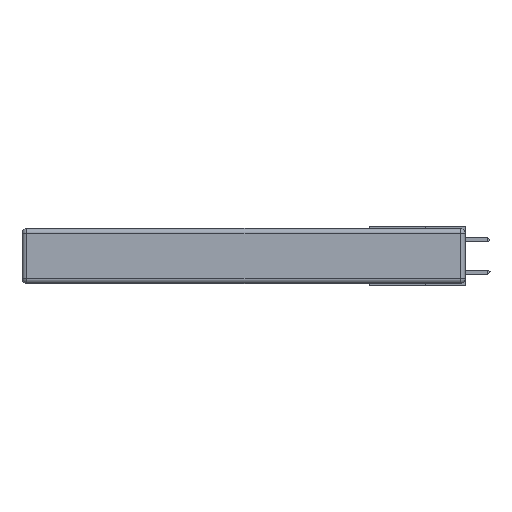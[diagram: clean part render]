
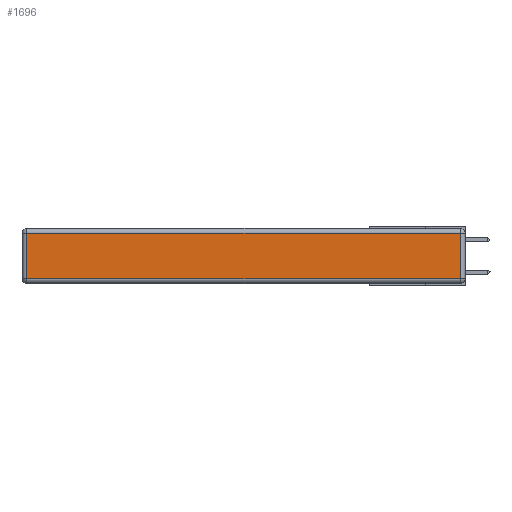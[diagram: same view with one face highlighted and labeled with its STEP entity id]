
A CAD part, left-side view. The second image highlights one B-rep face of the part: STEP entity #1696.
In plain terms, the highlighted planar face has unit normal (-1, 0, 0).
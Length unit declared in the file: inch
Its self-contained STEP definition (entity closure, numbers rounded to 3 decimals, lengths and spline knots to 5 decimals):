
#2 = DIRECTION ( 'NONE',  ( 0., 0., 1. ) ) ;
#451 = EDGE_CURVE ( 'NONE', #13760, #1633, #15265, .T. ) ;
#570 = LINE ( 'NONE', #2552, #5573 ) ;
#1633 = VERTEX_POINT ( 'NONE', #9276 ) ;
#1685 = DIRECTION ( 'NONE',  ( 0., -1., 0. ) ) ;
#1696 = ADVANCED_FACE ( 'NONE', ( #8168 ), #12979, .T. ) ;
#2439 = LINE ( 'NONE', #14198, #6668 ) ;
#2552 = CARTESIAN_POINT ( 'NONE',  ( 0., 2.72, -0.343 ) ) ;
#2918 = DIRECTION ( 'NONE',  ( 0., 1., 0. ) ) ;
#3330 = VERTEX_POINT ( 'NONE', #6634 ) ;
#5093 = LINE ( 'NONE', #8690, #9300 ) ;
#5573 = VECTOR ( 'NONE', #8496, 39.37008 ) ;
#5668 = EDGE_CURVE ( 'NONE', #1633, #10206, #2439, .T. ) ;
#5844 = DIRECTION ( 'NONE',  ( -1., 0., 0. ) ) ;
#6055 = ORIENTED_EDGE ( 'NONE', *, *, #5668, .T. ) ;
#6084 = EDGE_LOOP ( 'NONE', ( #11812, #6055, #13515, #13216 ) ) ;
#6634 = CARTESIAN_POINT ( 'NONE',  ( 0., 2.72, -0.03 ) ) ;
#6668 = VECTOR ( 'NONE', #7100, 39.37008 ) ;
#7100 = DIRECTION ( 'NONE',  ( 0., 0., 1. ) ) ;
#8168 = FACE_OUTER_BOUND ( 'NONE', #6084, .T. ) ;
#8496 = DIRECTION ( 'NONE',  ( 0., 0., -1. ) ) ;
#8575 = VECTOR ( 'NONE', #1685, 39.37008 ) ;
#8690 = CARTESIAN_POINT ( 'NONE',  ( 0., 2.75, -0.03 ) ) ;
#9276 = CARTESIAN_POINT ( 'NONE',  ( 0., 0.03, -0.313 ) ) ;
#9300 = VECTOR ( 'NONE', #2918, 39.37008 ) ;
#9401 = EDGE_CURVE ( 'NONE', #3330, #13760, #570, .T. ) ;
#10027 = CARTESIAN_POINT ( 'NONE',  ( 0., 2.72, -0.313 ) ) ;
#10206 = VERTEX_POINT ( 'NONE', #14999 ) ;
#11214 = CARTESIAN_POINT ( 'NONE',  ( 0., 0., -0.313 ) ) ;
#11812 = ORIENTED_EDGE ( 'NONE', *, *, #451, .T. ) ;
#11995 = EDGE_CURVE ( 'NONE', #10206, #3330, #5093, .T. ) ;
#12694 = AXIS2_PLACEMENT_3D ( 'NONE', #15272, #5844, #2 ) ;
#12979 = PLANE ( 'NONE',  #12694 ) ;
#13216 = ORIENTED_EDGE ( 'NONE', *, *, #9401, .T. ) ;
#13515 = ORIENTED_EDGE ( 'NONE', *, *, #11995, .T. ) ;
#13760 = VERTEX_POINT ( 'NONE', #10027 ) ;
#14198 = CARTESIAN_POINT ( 'NONE',  ( 0., 0.03, -0.343 ) ) ;
#14999 = CARTESIAN_POINT ( 'NONE',  ( 0., 0.03, -0.03 ) ) ;
#15265 = LINE ( 'NONE', #11214, #8575 ) ;
#15272 = CARTESIAN_POINT ( 'NONE',  ( 0., 0., -0.343 ) ) ;
